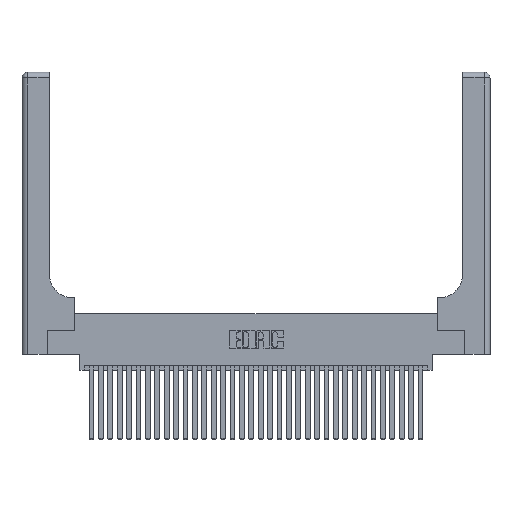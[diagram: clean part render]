
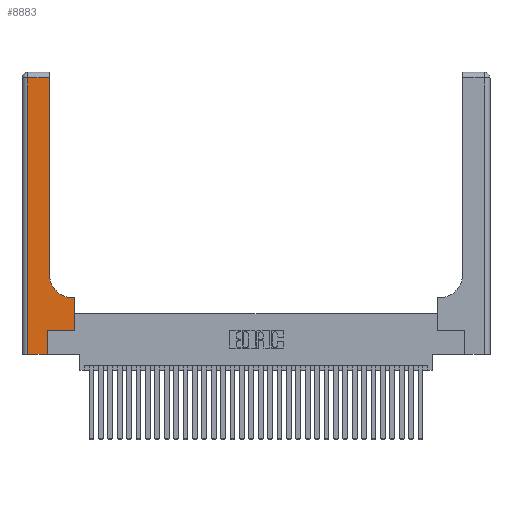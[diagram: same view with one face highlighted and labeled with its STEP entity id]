
A CAD part, top view. The second image highlights one B-rep face of the part: STEP entity #8883.
In plain terms, the highlighted planar face has unit normal (0, 0, 1).
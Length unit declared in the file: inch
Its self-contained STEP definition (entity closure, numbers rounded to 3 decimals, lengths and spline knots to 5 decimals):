
#326 = VERTEX_POINT ( 'NONE', #26327 ) ;
#1606 = CARTESIAN_POINT ( 'NONE',  ( 0.5415, 0.6, 0.37 ) ) ;
#1899 = CIRCLE ( 'NONE', #18842, 0.25 ) ;
#2125 = EDGE_CURVE ( 'NONE', #30655, #326, #1899, .T. ) ;
#2289 = VECTOR ( 'NONE', #33574, 39.37008 ) ;
#2441 = CARTESIAN_POINT ( 'NONE',  ( 0.269, 0.25, 0.37 ) ) ;
#2705 = VECTOR ( 'NONE', #18132, 39.37008 ) ;
#3325 = EDGE_LOOP ( 'NONE', ( #29326, #3517, #28866, #31957, #3716, #13016, #20032, #9076, #32443 ) ) ;
#3426 = LINE ( 'NONE', #6576, #23680 ) ;
#3517 = ORIENTED_EDGE ( 'NONE', *, *, #9415, .T. ) ;
#3716 = ORIENTED_EDGE ( 'NONE', *, *, #23938, .T. ) ;
#6576 = CARTESIAN_POINT ( 'NONE',  ( 0., 0., 0.37 ) ) ;
#7355 = CARTESIAN_POINT ( 'NONE',  ( 0., 2.94, 0.37 ) ) ;
#7721 = LINE ( 'NONE', #2441, #27505 ) ;
#8074 = FACE_OUTER_BOUND ( 'NONE', #3325, .T. ) ;
#8883 = ADVANCED_FACE ( 'NONE', ( #8074 ), #19476, .F. ) ;
#9011 = CARTESIAN_POINT ( 'NONE',  ( 0., 3., 0.37 ) ) ;
#9076 = ORIENTED_EDGE ( 'NONE', *, *, #10265, .T. ) ;
#9214 = CARTESIAN_POINT ( 'NONE',  ( 0.269, 0.25, 0.37 ) ) ;
#9365 = DIRECTION ( 'NONE',  ( 1., 0., 0. ) ) ;
#9366 = EDGE_CURVE ( 'NONE', #326, #32328, #32322, .T. ) ;
#9415 = EDGE_CURVE ( 'NONE', #32328, #21169, #16266, .T. ) ;
#9600 = DIRECTION ( 'NONE',  ( 0., 1., 0. ) ) ;
#10265 = EDGE_CURVE ( 'NONE', #23799, #30655, #13327, .T. ) ;
#10760 = CARTESIAN_POINT ( 'NONE',  ( 0.06, 2.94, 0.37 ) ) ;
#11736 = DIRECTION ( 'NONE',  ( -1., 0., 0. ) ) ;
#12110 = CARTESIAN_POINT ( 'NONE',  ( 0.5415, 0.85, 0.37 ) ) ;
#13016 = ORIENTED_EDGE ( 'NONE', *, *, #30250, .T. ) ;
#13327 = LINE ( 'NONE', #28078, #22375 ) ;
#14670 = DIRECTION ( 'NONE',  ( -1., 0., 0. ) ) ;
#14771 = DIRECTION ( 'NONE',  ( 0., 0., -1. ) ) ;
#14892 = EDGE_CURVE ( 'NONE', #33950, #28682, #3426, .T. ) ;
#16266 = LINE ( 'NONE', #7355, #29492 ) ;
#16333 = CARTESIAN_POINT ( 'NONE',  ( 0.269, 0., 0.37 ) ) ;
#17556 = DIRECTION ( 'NONE',  ( 1., 0., 0. ) ) ;
#18132 = DIRECTION ( 'NONE',  ( 0., 1., 0. ) ) ;
#18842 = AXIS2_PLACEMENT_3D ( 'NONE', #12110, #14771, #17556 ) ;
#19476 = PLANE ( 'NONE',  #28261 ) ;
#20032 = ORIENTED_EDGE ( 'NONE', *, *, #23689, .T. ) ;
#20354 = DIRECTION ( 'NONE',  ( -1., 0., 0. ) ) ;
#21169 = VERTEX_POINT ( 'NONE', #10760 ) ;
#21848 = DIRECTION ( 'NONE',  ( 0., 0., -1. ) ) ;
#22188 = CARTESIAN_POINT ( 'NONE',  ( 0.06, 0., 0.37 ) ) ;
#22375 = VECTOR ( 'NONE', #14670, 39.37008 ) ;
#23358 = LINE ( 'NONE', #33460, #2289 ) ;
#23680 = VECTOR ( 'NONE', #9365, 39.37008 ) ;
#23689 = EDGE_CURVE ( 'NONE', #29655, #23799, #28815, .T. ) ;
#23799 = VERTEX_POINT ( 'NONE', #29607 ) ;
#23938 = EDGE_CURVE ( 'NONE', #28682, #30001, #23358, .T. ) ;
#24128 = EDGE_CURVE ( 'NONE', #21169, #33950, #33711, .T. ) ;
#24204 = CARTESIAN_POINT ( 'NONE',  ( 0.5585, 0.25, 0.37 ) ) ;
#25977 = DIRECTION ( 'NONE',  ( 0., -1., 0. ) ) ;
#26143 = DIRECTION ( 'NONE',  ( 1., 0., 0. ) ) ;
#26327 = CARTESIAN_POINT ( 'NONE',  ( 0.2915, 0.85, 0.37 ) ) ;
#27505 = VECTOR ( 'NONE', #26143, 39.37008 ) ;
#27793 = CARTESIAN_POINT ( 'NONE',  ( 0.2915, 3., 0.37 ) ) ;
#28078 = CARTESIAN_POINT ( 'NONE',  ( 0.2915, 0.6, 0.37 ) ) ;
#28261 = AXIS2_PLACEMENT_3D ( 'NONE', #9011, #21848, #11736 ) ;
#28682 = VERTEX_POINT ( 'NONE', #16333 ) ;
#28709 = VECTOR ( 'NONE', #9600, 39.37008 ) ;
#28815 = LINE ( 'NONE', #33900, #2705 ) ;
#28866 = ORIENTED_EDGE ( 'NONE', *, *, #24128, .T. ) ;
#29326 = ORIENTED_EDGE ( 'NONE', *, *, #9366, .T. ) ;
#29492 = VECTOR ( 'NONE', #20354, 39.37008 ) ;
#29607 = CARTESIAN_POINT ( 'NONE',  ( 0.5585, 0.6, 0.37 ) ) ;
#29655 = VERTEX_POINT ( 'NONE', #24204 ) ;
#30001 = VERTEX_POINT ( 'NONE', #9214 ) ;
#30234 = CARTESIAN_POINT ( 'NONE',  ( 0.2915, 2.94, 0.37 ) ) ;
#30250 = EDGE_CURVE ( 'NONE', #30001, #29655, #7721, .T. ) ;
#30655 = VERTEX_POINT ( 'NONE', #1606 ) ;
#31359 = CARTESIAN_POINT ( 'NONE',  ( 0.06, 3., 0.37 ) ) ;
#31957 = ORIENTED_EDGE ( 'NONE', *, *, #14892, .T. ) ;
#32322 = LINE ( 'NONE', #27793, #28709 ) ;
#32328 = VERTEX_POINT ( 'NONE', #30234 ) ;
#32443 = ORIENTED_EDGE ( 'NONE', *, *, #2125, .T. ) ;
#33460 = CARTESIAN_POINT ( 'NONE',  ( 0.269, 0., 0.37 ) ) ;
#33574 = DIRECTION ( 'NONE',  ( 0., 1., 0. ) ) ;
#33711 = LINE ( 'NONE', #31359, #34101 ) ;
#33900 = CARTESIAN_POINT ( 'NONE',  ( 0.5585, 0.25, 0.37 ) ) ;
#33950 = VERTEX_POINT ( 'NONE', #22188 ) ;
#34101 = VECTOR ( 'NONE', #25977, 39.37008 ) ;
